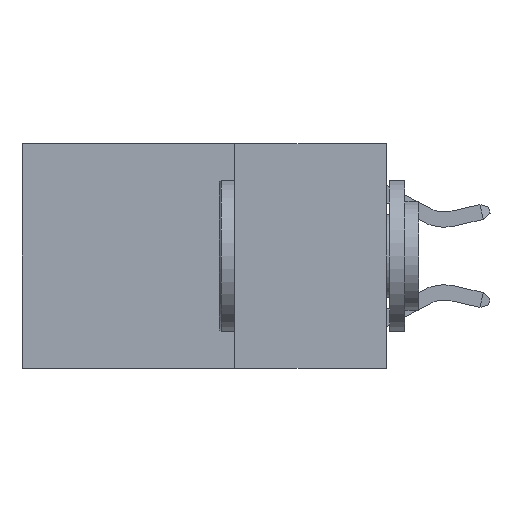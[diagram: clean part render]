
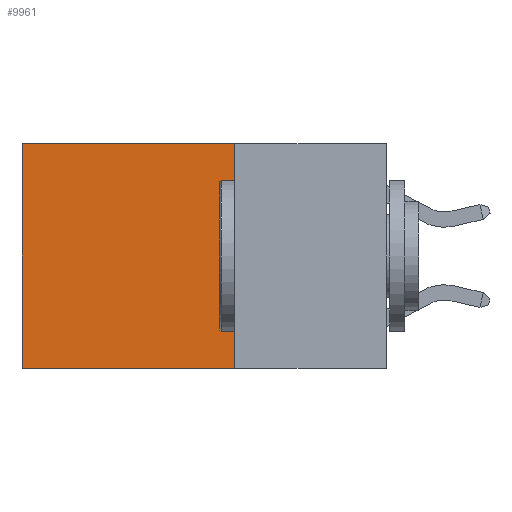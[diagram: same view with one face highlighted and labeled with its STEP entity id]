
A CAD part, left-side view. The second image highlights one B-rep face of the part: STEP entity #9961.
In plain terms, the highlighted planar face has unit normal (-1, 0, 0).
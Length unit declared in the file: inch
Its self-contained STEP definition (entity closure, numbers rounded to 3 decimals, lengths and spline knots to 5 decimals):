
#320 = DIRECTION ( 'NONE',  ( 1., 0., 0. ) ) ;
#1045 = DIRECTION ( 'NONE',  ( 0., 1., 0. ) ) ;
#1176 = FACE_OUTER_BOUND ( 'NONE', #7831, .T. ) ;
#1193 = VECTOR ( 'NONE', #9919, 39.37008 ) ;
#2401 = LINE ( 'NONE', #7910, #6508 ) ;
#2654 = VERTEX_POINT ( 'NONE', #12033 ) ;
#2705 = CARTESIAN_POINT ( 'NONE',  ( 0.2625, 0.25, 0. ) ) ;
#2959 = EDGE_CURVE ( 'NONE', #10313, #10691, #8201, .T. ) ;
#4066 = DIRECTION ( 'NONE',  ( 0., 0., -1. ) ) ;
#5277 = LINE ( 'NONE', #9512, #6960 ) ;
#5832 = CARTESIAN_POINT ( 'NONE',  ( 0.2625, 0.25, 0. ) ) ;
#6237 = CARTESIAN_POINT ( 'NONE',  ( 0.2625, 0.6, -0.37 ) ) ;
#6508 = VECTOR ( 'NONE', #1045, 39.37008 ) ;
#6641 = EDGE_CURVE ( 'NONE', #10313, #2654, #2401, .T. ) ;
#6960 = VECTOR ( 'NONE', #9768, 39.37008 ) ;
#7831 = EDGE_LOOP ( 'NONE', ( #15571, #13322, #8594, #15931 ) ) ;
#7910 = CARTESIAN_POINT ( 'NONE',  ( 0.2625, 0.25, 0. ) ) ;
#8201 = LINE ( 'NONE', #2705, #13468 ) ;
#8468 = LINE ( 'NONE', #14183, #1193 ) ;
#8530 = PLANE ( 'NONE',  #16370 ) ;
#8594 = ORIENTED_EDGE ( 'NONE', *, *, #2959, .F. ) ;
#9512 = CARTESIAN_POINT ( 'NONE',  ( 0.2625, 0.6, 0. ) ) ;
#9768 = DIRECTION ( 'NONE',  ( 0., 0., -1. ) ) ;
#9919 = DIRECTION ( 'NONE',  ( 0., 1., 0. ) ) ;
#9961 = ADVANCED_FACE ( 'NONE', ( #1176 ), #8530, .F. ) ;
#10313 = VERTEX_POINT ( 'NONE', #14962 ) ;
#10691 = VERTEX_POINT ( 'NONE', #17020 ) ;
#12033 = CARTESIAN_POINT ( 'NONE',  ( 0.2625, 0.6, 0. ) ) ;
#13322 = ORIENTED_EDGE ( 'NONE', *, *, #14299, .F. ) ;
#13468 = VECTOR ( 'NONE', #4066, 39.37008 ) ;
#14032 = VERTEX_POINT ( 'NONE', #6237 ) ;
#14183 = CARTESIAN_POINT ( 'NONE',  ( 0.2625, 0.25, -0.37 ) ) ;
#14299 = EDGE_CURVE ( 'NONE', #10691, #14032, #8468, .T. ) ;
#14962 = CARTESIAN_POINT ( 'NONE',  ( 0.2625, 0.25, 0. ) ) ;
#15096 = DIRECTION ( 'NONE',  ( 0., 0., -1. ) ) ;
#15571 = ORIENTED_EDGE ( 'NONE', *, *, #15885, .T. ) ;
#15885 = EDGE_CURVE ( 'NONE', #2654, #14032, #5277, .T. ) ;
#15931 = ORIENTED_EDGE ( 'NONE', *, *, #6641, .T. ) ;
#16370 = AXIS2_PLACEMENT_3D ( 'NONE', #5832, #320, #15096 ) ;
#17020 = CARTESIAN_POINT ( 'NONE',  ( 0.2625, 0.25, -0.37 ) ) ;
